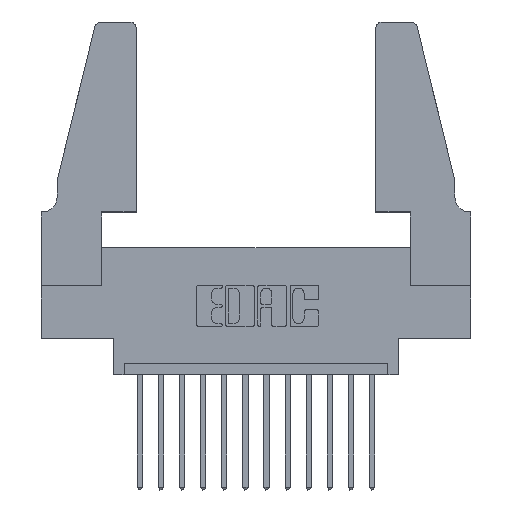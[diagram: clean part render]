
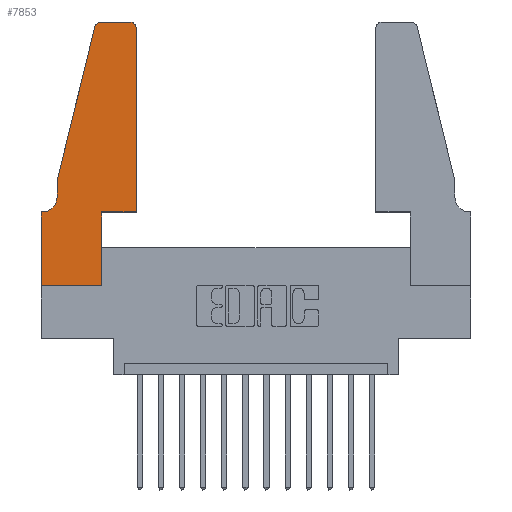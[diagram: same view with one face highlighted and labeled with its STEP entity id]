
A CAD part, top view. The second image highlights one B-rep face of the part: STEP entity #7853.
In plain terms, the highlighted planar face has unit normal (0, 0, 1).
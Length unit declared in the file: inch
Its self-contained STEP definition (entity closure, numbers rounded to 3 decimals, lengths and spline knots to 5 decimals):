
#196 = EDGE_CURVE ( 'NONE', #470, #11716, #5470, .T. ) ;
#273 = DIRECTION ( 'NONE',  ( 0., 0., 1. ) ) ;
#470 = VERTEX_POINT ( 'NONE', #11136 ) ;
#491 = EDGE_CURVE ( 'NONE', #6275, #8091, #15024, .T. ) ;
#697 = CARTESIAN_POINT ( 'NONE',  ( 0.0755, 0.35, 0.37 ) ) ;
#723 = ORIENTED_EDGE ( 'NONE', *, *, #7466, .T. ) ;
#775 = LINE ( 'NONE', #697, #9163 ) ;
#833 = EDGE_CURVE ( 'NONE', #14408, #4290, #6921, .T. ) ;
#946 = VECTOR ( 'NONE', #13962, 39.37008 ) ;
#1143 = CARTESIAN_POINT ( 'NONE',  ( 0.0055, 0.35, 0.37 ) ) ;
#1437 = EDGE_LOOP ( 'NONE', ( #6810, #13987, #10359, #11151, #3070, #3761, #723, #11654, #9401, #4991, #8996, #8250 ) ) ;
#1531 = CARTESIAN_POINT ( 'NONE',  ( 0.2865, 0.35, 0.37 ) ) ;
#1562 = FACE_OUTER_BOUND ( 'NONE', #1437, .T. ) ;
#2242 = AXIS2_PLACEMENT_3D ( 'NONE', #5304, #4689, #4640 ) ;
#2746 = VERTEX_POINT ( 'NONE', #7759 ) ;
#2778 = CARTESIAN_POINT ( 'NONE',  ( 0.2605, 1.25, 0.37 ) ) ;
#2878 = DIRECTION ( 'NONE',  ( 0., 1., 0. ) ) ;
#3070 = ORIENTED_EDGE ( 'NONE', *, *, #5451, .T. ) ;
#3467 = CARTESIAN_POINT ( 'NONE',  ( 0., 0., 0.37 ) ) ;
#3761 = ORIENTED_EDGE ( 'NONE', *, *, #8732, .T. ) ;
#3871 = AXIS2_PLACEMENT_3D ( 'NONE', #13174, #273, #4948 ) ;
#3894 = EDGE_CURVE ( 'NONE', #9052, #14664, #11096, .T. ) ;
#4243 = CARTESIAN_POINT ( 'NONE',  ( 0.0755, 0.42, 0.37 ) ) ;
#4274 = CARTESIAN_POINT ( 'NONE',  ( 0., 0., 0.37 ) ) ;
#4290 = VERTEX_POINT ( 'NONE', #12125 ) ;
#4640 = DIRECTION ( 'NONE',  ( 1., 0., 0. ) ) ;
#4689 = DIRECTION ( 'NONE',  ( 0., 0., 1. ) ) ;
#4948 = DIRECTION ( 'NONE',  ( 1., 0., 0. ) ) ;
#4991 = ORIENTED_EDGE ( 'NONE', *, *, #196, .T. ) ;
#5087 = EDGE_CURVE ( 'NONE', #2746, #9052, #12448, .T. ) ;
#5147 = LINE ( 'NONE', #4274, #14571 ) ;
#5304 = CARTESIAN_POINT ( 'NONE',  ( 0., 0.35, 0.37 ) ) ;
#5338 = CARTESIAN_POINT ( 'NONE',  ( 0., 0.35, 0.37 ) ) ;
#5450 = CARTESIAN_POINT ( 'NONE',  ( 0.2865, 0., 0.37 ) ) ;
#5451 = EDGE_CURVE ( 'NONE', #10438, #14140, #14974, .T. ) ;
#5465 = DIRECTION ( 'NONE',  ( 0., -1., 0. ) ) ;
#5470 = LINE ( 'NONE', #12765, #946 ) ;
#5528 = DIRECTION ( 'NONE',  ( -1., 0., 0. ) ) ;
#5875 = CARTESIAN_POINT ( 'NONE',  ( 0.4505, 0.35, 0.37 ) ) ;
#5934 = AXIS2_PLACEMENT_3D ( 'NONE', #12074, #11966, #7347 ) ;
#6201 = LINE ( 'NONE', #14163, #13442 ) ;
#6275 = VERTEX_POINT ( 'NONE', #3467 ) ;
#6810 = ORIENTED_EDGE ( 'NONE', *, *, #3894, .T. ) ;
#6826 = DIRECTION ( 'NONE',  ( -0.239, -0.971, 0. ) ) ;
#6921 = LINE ( 'NONE', #12631, #13020 ) ;
#6986 = CIRCLE ( 'NONE', #3871, 0.03 ) ;
#7182 = VECTOR ( 'NONE', #9806, 39.37008 ) ;
#7302 = DIRECTION ( 'NONE',  ( 1., 0., 0. ) ) ;
#7332 = LINE ( 'NONE', #15345, #9009 ) ;
#7347 = DIRECTION ( 'NONE',  ( -1., 0., 0. ) ) ;
#7466 = EDGE_CURVE ( 'NONE', #12678, #6275, #5147, .T. ) ;
#7710 = EDGE_CURVE ( 'NONE', #14664, #14408, #6986, .T. ) ;
#7759 = CARTESIAN_POINT ( 'NONE',  ( 0.4505, 1.22, 0.37 ) ) ;
#7853 = ADVANCED_FACE ( 'NONE', ( #1562 ), #12413, .T. ) ;
#7972 = DIRECTION ( 'NONE',  ( 1., 0., 0. ) ) ;
#7981 = EDGE_CURVE ( 'NONE', #8091, #470, #12555, .T. ) ;
#8091 = VERTEX_POINT ( 'NONE', #5450 ) ;
#8214 = EDGE_CURVE ( 'NONE', #11716, #2746, #7332, .T. ) ;
#8230 = DIRECTION ( 'NONE',  ( 0., -1., 0. ) ) ;
#8250 = ORIENTED_EDGE ( 'NONE', *, *, #5087, .T. ) ;
#8619 = VECTOR ( 'NONE', #2878, 39.37008 ) ;
#8732 = EDGE_CURVE ( 'NONE', #14140, #12678, #775, .T. ) ;
#8966 = CARTESIAN_POINT ( 'NONE',  ( 0.4205, 1.22, 0.37 ) ) ;
#8996 = ORIENTED_EDGE ( 'NONE', *, *, #8214, .T. ) ;
#9009 = VECTOR ( 'NONE', #9743, 39.37008 ) ;
#9052 = VERTEX_POINT ( 'NONE', #10658 ) ;
#9163 = VECTOR ( 'NONE', #5528, 39.37008 ) ;
#9401 = ORIENTED_EDGE ( 'NONE', *, *, #7981, .T. ) ;
#9743 = DIRECTION ( 'NONE',  ( 0., 1., 0. ) ) ;
#9806 = DIRECTION ( 'NONE',  ( -1., 0., 0. ) ) ;
#10359 = ORIENTED_EDGE ( 'NONE', *, *, #833, .T. ) ;
#10438 = VERTEX_POINT ( 'NONE', #4243 ) ;
#10658 = CARTESIAN_POINT ( 'NONE',  ( 0.4205, 1.25, 0.37 ) ) ;
#10838 = CARTESIAN_POINT ( 'NONE',  ( 0.284, 1.25, 0.37 ) ) ;
#11096 = LINE ( 'NONE', #2778, #7182 ) ;
#11136 = CARTESIAN_POINT ( 'NONE',  ( 0.2865, 0.35, 0.37 ) ) ;
#11151 = ORIENTED_EDGE ( 'NONE', *, *, #13562, .T. ) ;
#11654 = ORIENTED_EDGE ( 'NONE', *, *, #491, .T. ) ;
#11716 = VERTEX_POINT ( 'NONE', #5875 ) ;
#11966 = DIRECTION ( 'NONE',  ( 0., 0., -1. ) ) ;
#12074 = CARTESIAN_POINT ( 'NONE',  ( 0.0055, 0.42, 0.37 ) ) ;
#12101 = CARTESIAN_POINT ( 'NONE',  ( 0.25487, 1.22718, 0.37 ) ) ;
#12125 = CARTESIAN_POINT ( 'NONE',  ( 0.0755, 0.5, 0.37 ) ) ;
#12413 = PLANE ( 'NONE',  #2242 ) ;
#12448 = CIRCLE ( 'NONE', #14738, 0.03 ) ;
#12555 = LINE ( 'NONE', #1531, #8619 ) ;
#12631 = CARTESIAN_POINT ( 'NONE',  ( 0.0755, 0.5, 0.37 ) ) ;
#12678 = VERTEX_POINT ( 'NONE', #5338 ) ;
#12765 = CARTESIAN_POINT ( 'NONE',  ( 0.4505, 0.35, 0.37 ) ) ;
#12864 = VECTOR ( 'NONE', #7972, 39.37008 ) ;
#13020 = VECTOR ( 'NONE', #6826, 39.37008 ) ;
#13174 = CARTESIAN_POINT ( 'NONE',  ( 0.284, 1.22, 0.37 ) ) ;
#13391 = DIRECTION ( 'NONE',  ( 0., 0., 1. ) ) ;
#13442 = VECTOR ( 'NONE', #8230, 39.37008 ) ;
#13562 = EDGE_CURVE ( 'NONE', #4290, #10438, #6201, .T. ) ;
#13962 = DIRECTION ( 'NONE',  ( 1., 0., 0. ) ) ;
#13987 = ORIENTED_EDGE ( 'NONE', *, *, #7710, .T. ) ;
#14140 = VERTEX_POINT ( 'NONE', #1143 ) ;
#14163 = CARTESIAN_POINT ( 'NONE',  ( 0.0755, 0.5, 0.37 ) ) ;
#14408 = VERTEX_POINT ( 'NONE', #12101 ) ;
#14571 = VECTOR ( 'NONE', #5465, 39.37008 ) ;
#14664 = VERTEX_POINT ( 'NONE', #10838 ) ;
#14738 = AXIS2_PLACEMENT_3D ( 'NONE', #8966, #13391, #7302 ) ;
#14974 = CIRCLE ( 'NONE', #5934, 0.07 ) ;
#15024 = LINE ( 'NONE', #15132, #12864 ) ;
#15132 = CARTESIAN_POINT ( 'NONE',  ( 0., 0., 0.37 ) ) ;
#15345 = CARTESIAN_POINT ( 'NONE',  ( 0.4505, 0.35, 0.37 ) ) ;
